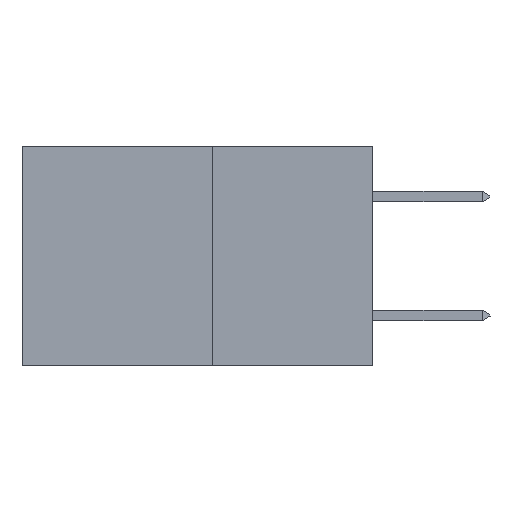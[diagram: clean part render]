
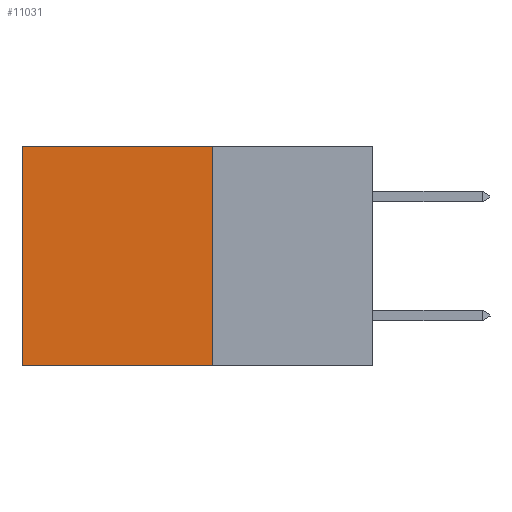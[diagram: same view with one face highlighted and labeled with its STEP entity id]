
A CAD part, left-side view. The second image highlights one B-rep face of the part: STEP entity #11031.
In plain terms, the highlighted planar face has unit normal (-1, 0, 0).
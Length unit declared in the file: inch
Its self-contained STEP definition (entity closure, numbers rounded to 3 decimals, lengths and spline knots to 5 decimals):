
#405 = PLANE ( 'NONE',  #2440 ) ;
#764 = DIRECTION ( 'NONE',  ( 0., 0., -1. ) ) ;
#859 = CARTESIAN_POINT ( 'NONE',  ( 0.277, 0.27, 0. ) ) ;
#991 = CARTESIAN_POINT ( 'NONE',  ( 0.277, 0.27, 0. ) ) ;
#1124 = LINE ( 'NONE', #991, #8084 ) ;
#1279 = ORIENTED_EDGE ( 'NONE', *, *, #3235, .F. ) ;
#1283 = DIRECTION ( 'NONE',  ( 0., 1., 0. ) ) ;
#1400 = ORIENTED_EDGE ( 'NONE', *, *, #8365, .T. ) ;
#1449 = ORIENTED_EDGE ( 'NONE', *, *, #4303, .F. ) ;
#1720 = VECTOR ( 'NONE', #1283, 39.37008 ) ;
#2209 = FACE_OUTER_BOUND ( 'NONE', #7652, .T. ) ;
#2440 = AXIS2_PLACEMENT_3D ( 'NONE', #4865, #9903, #4896 ) ;
#3235 = EDGE_CURVE ( 'NONE', #3611, #6914, #4139, .T. ) ;
#3379 = DIRECTION ( 'NONE',  ( 0., 0., -1. ) ) ;
#3611 = VERTEX_POINT ( 'NONE', #6003 ) ;
#3632 = EDGE_CURVE ( 'NONE', #9017, #6914, #7594, .T. ) ;
#3813 = CARTESIAN_POINT ( 'NONE',  ( 0.277, 0.59, 0. ) ) ;
#4139 = LINE ( 'NONE', #7049, #1720 ) ;
#4303 = EDGE_CURVE ( 'NONE', #6487, #3611, #10770, .T. ) ;
#4865 = CARTESIAN_POINT ( 'NONE',  ( 0.277, 0.27, -0.37 ) ) ;
#4896 = DIRECTION ( 'NONE',  ( 0., 0., -1. ) ) ;
#5231 = CARTESIAN_POINT ( 'NONE',  ( 0.277, 0.27, -0.37 ) ) ;
#5950 = ORIENTED_EDGE ( 'NONE', *, *, #3632, .T. ) ;
#6003 = CARTESIAN_POINT ( 'NONE',  ( 0.277, 0.27, -0.37 ) ) ;
#6487 = VERTEX_POINT ( 'NONE', #859 ) ;
#6914 = VERTEX_POINT ( 'NONE', #10120 ) ;
#7049 = CARTESIAN_POINT ( 'NONE',  ( 0.277, 0.27, -0.37 ) ) ;
#7117 = DIRECTION ( 'NONE',  ( 0., 1., 0. ) ) ;
#7594 = LINE ( 'NONE', #9304, #10047 ) ;
#7652 = EDGE_LOOP ( 'NONE', ( #5950, #1279, #1449, #1400 ) ) ;
#8084 = VECTOR ( 'NONE', #7117, 39.37008 ) ;
#8365 = EDGE_CURVE ( 'NONE', #6487, #9017, #1124, .T. ) ;
#8596 = VECTOR ( 'NONE', #764, 39.37008 ) ;
#9017 = VERTEX_POINT ( 'NONE', #3813 ) ;
#9304 = CARTESIAN_POINT ( 'NONE',  ( 0.277, 0.59, -0.37 ) ) ;
#9903 = DIRECTION ( 'NONE',  ( 1., 0., 0. ) ) ;
#10047 = VECTOR ( 'NONE', #3379, 39.37008 ) ;
#10120 = CARTESIAN_POINT ( 'NONE',  ( 0.277, 0.59, -0.37 ) ) ;
#10770 = LINE ( 'NONE', #5231, #8596 ) ;
#11031 = ADVANCED_FACE ( 'NONE', ( #2209 ), #405, .F. ) ;
